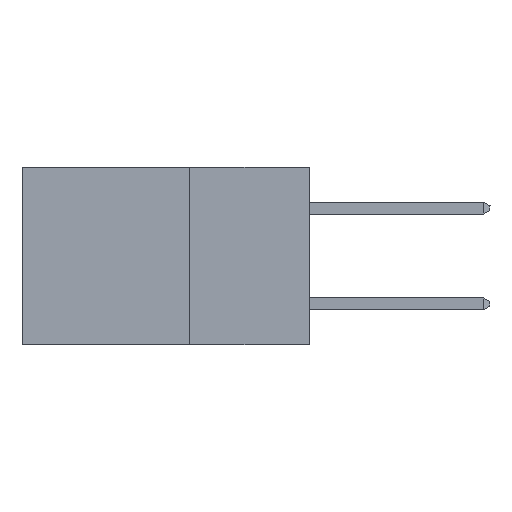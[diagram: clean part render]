
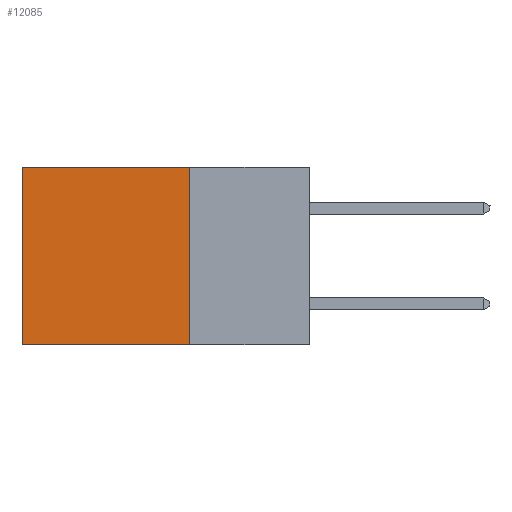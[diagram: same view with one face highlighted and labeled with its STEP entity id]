
A CAD part, left-side view. The second image highlights one B-rep face of the part: STEP entity #12085.
In plain terms, the highlighted planar face has unit normal (-1, 0, 0).
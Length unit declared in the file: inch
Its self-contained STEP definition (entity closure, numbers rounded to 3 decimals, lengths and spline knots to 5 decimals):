
#408 = LINE ( 'NONE', #12826, #5524 ) ;
#691 = DIRECTION ( 'NONE',  ( 0., 1., 0. ) ) ;
#1022 = VECTOR ( 'NONE', #2179, 39.37008 ) ;
#1206 = EDGE_CURVE ( 'NONE', #5637, #2450, #10022, .T. ) ;
#1347 = PLANE ( 'NONE',  #3488 ) ;
#1817 = FACE_OUTER_BOUND ( 'NONE', #4317, .T. ) ;
#1953 = CARTESIAN_POINT ( 'NONE',  ( 0.2875, 0.6, -0.37 ) ) ;
#2179 = DIRECTION ( 'NONE',  ( 0., 1., 0. ) ) ;
#2450 = VERTEX_POINT ( 'NONE', #5453 ) ;
#2906 = EDGE_CURVE ( 'NONE', #5637, #8218, #408, .T. ) ;
#3247 = VECTOR ( 'NONE', #691, 39.37008 ) ;
#3398 = ORIENTED_EDGE ( 'NONE', *, *, #13636, .F. ) ;
#3488 = AXIS2_PLACEMENT_3D ( 'NONE', #4876, #7167, #3743 ) ;
#3743 = DIRECTION ( 'NONE',  ( 0., 0., -1. ) ) ;
#3777 = CARTESIAN_POINT ( 'NONE',  ( 0.2875, 0.6, 0. ) ) ;
#3908 = ORIENTED_EDGE ( 'NONE', *, *, #1206, .T. ) ;
#4317 = EDGE_LOOP ( 'NONE', ( #14218, #3398, #11828, #3908 ) ) ;
#4336 = CARTESIAN_POINT ( 'NONE',  ( 0.2875, 0.25, -0.37 ) ) ;
#4876 = CARTESIAN_POINT ( 'NONE',  ( 0.2875, 0.25, 0. ) ) ;
#5453 = CARTESIAN_POINT ( 'NONE',  ( 0.2875, 0.6, 0. ) ) ;
#5524 = VECTOR ( 'NONE', #9350, 39.37008 ) ;
#5637 = VERTEX_POINT ( 'NONE', #9612 ) ;
#5951 = DIRECTION ( 'NONE',  ( 0., 0., -1. ) ) ;
#6360 = LINE ( 'NONE', #4336, #3247 ) ;
#7167 = DIRECTION ( 'NONE',  ( 1., 0., 0. ) ) ;
#8218 = VERTEX_POINT ( 'NONE', #9739 ) ;
#9350 = DIRECTION ( 'NONE',  ( 0., 0., -1. ) ) ;
#9612 = CARTESIAN_POINT ( 'NONE',  ( 0.2875, 0.25, 0. ) ) ;
#9739 = CARTESIAN_POINT ( 'NONE',  ( 0.2875, 0.25, -0.37 ) ) ;
#10022 = LINE ( 'NONE', #13935, #1022 ) ;
#11733 = LINE ( 'NONE', #3777, #15290 ) ;
#11828 = ORIENTED_EDGE ( 'NONE', *, *, #2906, .F. ) ;
#12085 = ADVANCED_FACE ( 'NONE', ( #1817 ), #1347, .F. ) ;
#12519 = VERTEX_POINT ( 'NONE', #1953 ) ;
#12826 = CARTESIAN_POINT ( 'NONE',  ( 0.2875, 0.25, 0. ) ) ;
#13302 = EDGE_CURVE ( 'NONE', #2450, #12519, #11733, .T. ) ;
#13636 = EDGE_CURVE ( 'NONE', #8218, #12519, #6360, .T. ) ;
#13935 = CARTESIAN_POINT ( 'NONE',  ( 0.2875, 0.25, 0. ) ) ;
#14218 = ORIENTED_EDGE ( 'NONE', *, *, #13302, .T. ) ;
#15290 = VECTOR ( 'NONE', #5951, 39.37008 ) ;
